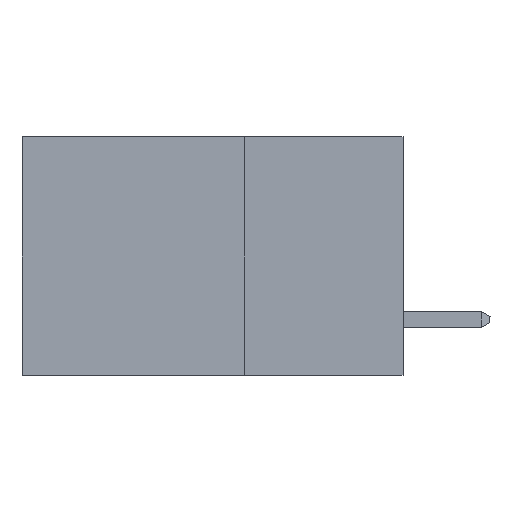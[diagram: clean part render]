
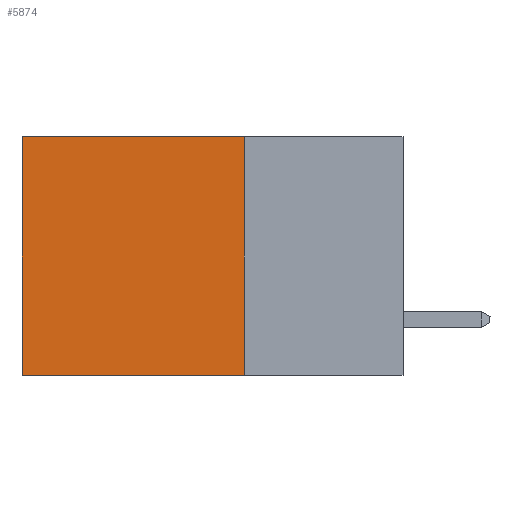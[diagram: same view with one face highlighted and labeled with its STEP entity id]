
A CAD part, left-side view. The second image highlights one B-rep face of the part: STEP entity #5874.
In plain terms, the highlighted planar face has unit normal (-1, 0, 0).
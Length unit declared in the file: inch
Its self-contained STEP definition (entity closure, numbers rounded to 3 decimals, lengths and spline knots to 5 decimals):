
#178 = FACE_OUTER_BOUND ( 'NONE', #1993, .T. ) ;
#737 = CARTESIAN_POINT ( 'NONE',  ( 0.2875, 0.25, -0.375 ) ) ;
#1491 = DIRECTION ( 'NONE',  ( 0., 1., 0. ) ) ;
#1993 = EDGE_LOOP ( 'NONE', ( #8494, #14430, #7295, #8281 ) ) ;
#2169 = CARTESIAN_POINT ( 'NONE',  ( 0.2875, 0.25, 0. ) ) ;
#2200 = DIRECTION ( 'NONE',  ( 1., 0., 0. ) ) ;
#2297 = DIRECTION ( 'NONE',  ( 0., 0., -1. ) ) ;
#2587 = CARTESIAN_POINT ( 'NONE',  ( 0.2875, 0.25, -0.375 ) ) ;
#2940 = VERTEX_POINT ( 'NONE', #6125 ) ;
#3335 = LINE ( 'NONE', #5102, #5530 ) ;
#3458 = CARTESIAN_POINT ( 'NONE',  ( 0.2875, 0.25, -0.375 ) ) ;
#3875 = EDGE_CURVE ( 'NONE', #10487, #2940, #9958, .T. ) ;
#4086 = LINE ( 'NONE', #2587, #11023 ) ;
#4433 = DIRECTION ( 'NONE',  ( 0., 1., 0. ) ) ;
#4572 = AXIS2_PLACEMENT_3D ( 'NONE', #3458, #2200, #2297 ) ;
#5102 = CARTESIAN_POINT ( 'NONE',  ( 0.2875, 0.6, -0.375 ) ) ;
#5530 = VECTOR ( 'NONE', #12002, 39.37008 ) ;
#5714 = VECTOR ( 'NONE', #1491, 39.37008 ) ;
#5817 = VERTEX_POINT ( 'NONE', #14014 ) ;
#5874 = ADVANCED_FACE ( 'NONE', ( #178 ), #8032, .F. ) ;
#6125 = CARTESIAN_POINT ( 'NONE',  ( 0.2875, 0.6, 0. ) ) ;
#7295 = ORIENTED_EDGE ( 'NONE', *, *, #11233, .F. ) ;
#7367 = DIRECTION ( 'NONE',  ( 0., 0., -1. ) ) ;
#8032 = PLANE ( 'NONE',  #4572 ) ;
#8133 = EDGE_CURVE ( 'NONE', #10221, #5817, #9001, .T. ) ;
#8281 = ORIENTED_EDGE ( 'NONE', *, *, #3875, .T. ) ;
#8315 = VECTOR ( 'NONE', #4433, 39.37008 ) ;
#8494 = ORIENTED_EDGE ( 'NONE', *, *, #12158, .T. ) ;
#9001 = LINE ( 'NONE', #12959, #5714 ) ;
#9958 = LINE ( 'NONE', #14852, #8315 ) ;
#10221 = VERTEX_POINT ( 'NONE', #737 ) ;
#10487 = VERTEX_POINT ( 'NONE', #2169 ) ;
#11023 = VECTOR ( 'NONE', #7367, 39.37008 ) ;
#11233 = EDGE_CURVE ( 'NONE', #10487, #10221, #4086, .T. ) ;
#12002 = DIRECTION ( 'NONE',  ( 0., 0., -1. ) ) ;
#12158 = EDGE_CURVE ( 'NONE', #2940, #5817, #3335, .T. ) ;
#12959 = CARTESIAN_POINT ( 'NONE',  ( 0.2875, 0.25, -0.375 ) ) ;
#14014 = CARTESIAN_POINT ( 'NONE',  ( 0.2875, 0.6, -0.375 ) ) ;
#14430 = ORIENTED_EDGE ( 'NONE', *, *, #8133, .F. ) ;
#14852 = CARTESIAN_POINT ( 'NONE',  ( 0.2875, 0.25, 0. ) ) ;
